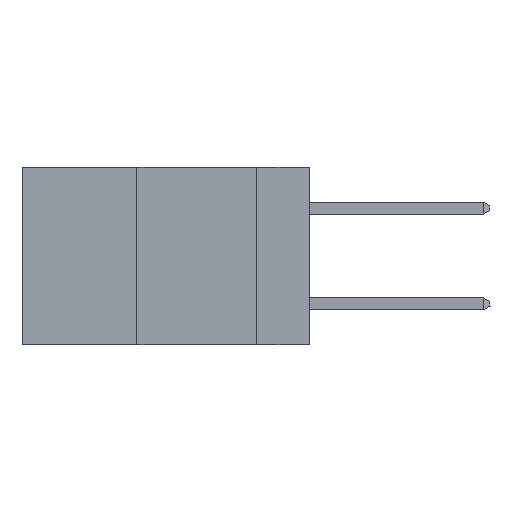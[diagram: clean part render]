
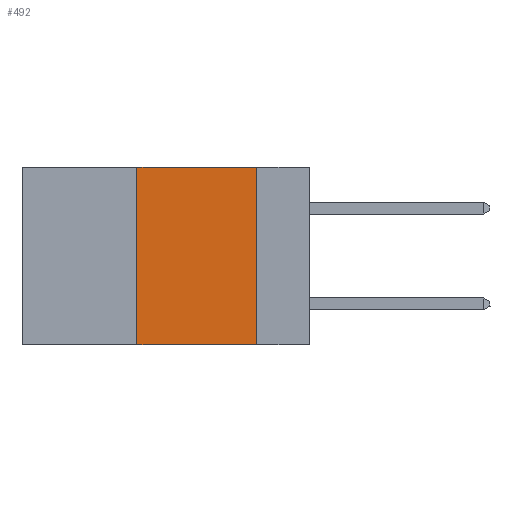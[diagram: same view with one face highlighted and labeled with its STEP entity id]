
A CAD part, left-side view. The second image highlights one B-rep face of the part: STEP entity #492.
In plain terms, the highlighted planar face has unit normal (-1, 0, 0).
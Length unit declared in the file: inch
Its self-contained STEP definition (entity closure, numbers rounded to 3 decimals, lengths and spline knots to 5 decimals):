
#2 = CARTESIAN_POINT ( 'NONE',  ( 0., 0.36, -0.37 ) ) ;
#396 = PLANE ( 'NONE',  #6921 ) ;
#492 = ADVANCED_FACE ( 'NONE', ( #8367 ), #396, .F. ) ;
#630 = LINE ( 'NONE', #10112, #7651 ) ;
#993 = VERTEX_POINT ( 'NONE', #2 ) ;
#1827 = LINE ( 'NONE', #5373, #4662 ) ;
#2057 = CARTESIAN_POINT ( 'NONE',  ( 0., 0.36, 0. ) ) ;
#2076 = CARTESIAN_POINT ( 'NONE',  ( 0., 0.11, 0. ) ) ;
#3322 = EDGE_LOOP ( 'NONE', ( #10179, #7812, #7788, #4300 ) ) ;
#3751 = EDGE_CURVE ( 'NONE', #4825, #4507, #6520, .T. ) ;
#4171 = DIRECTION ( 'NONE',  ( 0., -1., 0. ) ) ;
#4300 = ORIENTED_EDGE ( 'NONE', *, *, #4584, .T. ) ;
#4505 = DIRECTION ( 'NONE',  ( 0., -1., 0. ) ) ;
#4507 = VERTEX_POINT ( 'NONE', #6000 ) ;
#4584 = EDGE_CURVE ( 'NONE', #993, #4507, #1827, .T. ) ;
#4662 = VECTOR ( 'NONE', #4505, 39.37008 ) ;
#4802 = CARTESIAN_POINT ( 'NONE',  ( 0., 0.6, 0. ) ) ;
#4825 = VERTEX_POINT ( 'NONE', #9755 ) ;
#4951 = LINE ( 'NONE', #2057, #10968 ) ;
#5373 = CARTESIAN_POINT ( 'NONE',  ( 0., 0.6, -0.37 ) ) ;
#5451 = EDGE_CURVE ( 'NONE', #8625, #4825, #630, .T. ) ;
#5610 = DIRECTION ( 'NONE',  ( 1., 0., 0. ) ) ;
#6000 = CARTESIAN_POINT ( 'NONE',  ( 0., 0.11, -0.37 ) ) ;
#6281 = VECTOR ( 'NONE', #10938, 39.37008 ) ;
#6336 = EDGE_CURVE ( 'NONE', #993, #8625, #4951, .T. ) ;
#6502 = DIRECTION ( 'NONE',  ( 0., 0., 1. ) ) ;
#6520 = LINE ( 'NONE', #2076, #6281 ) ;
#6921 = AXIS2_PLACEMENT_3D ( 'NONE', #4802, #5610, #8486 ) ;
#6936 = CARTESIAN_POINT ( 'NONE',  ( 0., 0.36, 0. ) ) ;
#7651 = VECTOR ( 'NONE', #4171, 39.37008 ) ;
#7788 = ORIENTED_EDGE ( 'NONE', *, *, #6336, .F. ) ;
#7812 = ORIENTED_EDGE ( 'NONE', *, *, #5451, .F. ) ;
#8367 = FACE_OUTER_BOUND ( 'NONE', #3322, .T. ) ;
#8486 = DIRECTION ( 'NONE',  ( 0., 0., -1. ) ) ;
#8625 = VERTEX_POINT ( 'NONE', #6936 ) ;
#9755 = CARTESIAN_POINT ( 'NONE',  ( 0., 0.11, 0. ) ) ;
#10112 = CARTESIAN_POINT ( 'NONE',  ( 0., 0.6, 0. ) ) ;
#10179 = ORIENTED_EDGE ( 'NONE', *, *, #3751, .F. ) ;
#10938 = DIRECTION ( 'NONE',  ( 0., 0., -1. ) ) ;
#10968 = VECTOR ( 'NONE', #6502, 39.37008 ) ;
